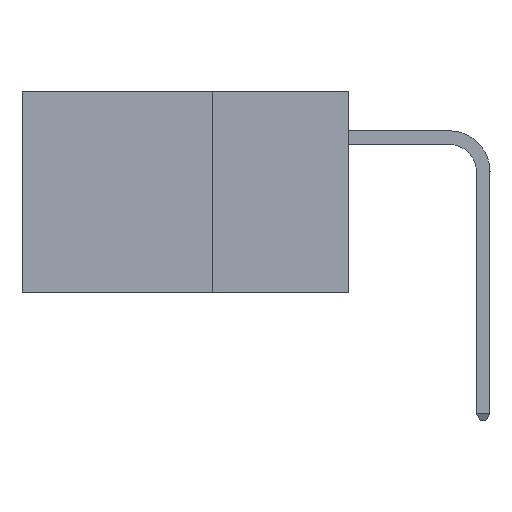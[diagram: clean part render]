
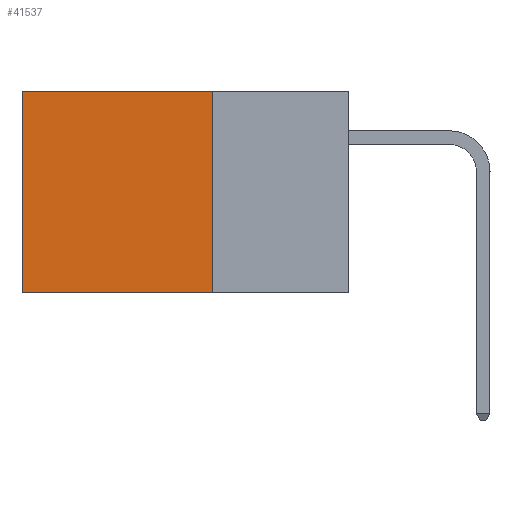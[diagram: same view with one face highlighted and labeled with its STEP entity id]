
A CAD part, left-side view. The second image highlights one B-rep face of the part: STEP entity #41537.
In plain terms, the highlighted planar face has unit normal (-1, 0, 0).
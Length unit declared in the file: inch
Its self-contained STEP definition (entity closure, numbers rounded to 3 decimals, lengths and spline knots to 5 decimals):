
#306 = ORIENTED_EDGE ( 'NONE', *, *, #25987, .F. ) ;
#321 = EDGE_CURVE ( 'NONE', #9929, #9612, #21247, .T. ) ;
#1148 = CARTESIAN_POINT ( 'NONE',  ( 0.2875, 0.25, 0. ) ) ;
#2748 = CARTESIAN_POINT ( 'NONE',  ( 0.2875, 0.6, 0. ) ) ;
#3598 = FACE_OUTER_BOUND ( 'NONE', #4497, .T. ) ;
#4399 = LINE ( 'NONE', #32380, #9884 ) ;
#4497 = EDGE_LOOP ( 'NONE', ( #27915, #306, #9105, #9770 ) ) ;
#5190 = CARTESIAN_POINT ( 'NONE',  ( 0.2875, 0.6, -0.37 ) ) ;
#6873 = VERTEX_POINT ( 'NONE', #39165 ) ;
#7708 = DIRECTION ( 'NONE',  ( 0., 0., -1. ) ) ;
#9105 = ORIENTED_EDGE ( 'NONE', *, *, #31277, .F. ) ;
#9612 = VERTEX_POINT ( 'NONE', #5190 ) ;
#9770 = ORIENTED_EDGE ( 'NONE', *, *, #43562, .T. ) ;
#9884 = VECTOR ( 'NONE', #39561, 39.37008 ) ;
#9929 = VERTEX_POINT ( 'NONE', #41348 ) ;
#13336 = VECTOR ( 'NONE', #37983, 39.37008 ) ;
#14070 = DIRECTION ( 'NONE',  ( 0., 0., -1. ) ) ;
#14296 = VECTOR ( 'NONE', #19797, 39.37008 ) ;
#14437 = PLANE ( 'NONE',  #30230 ) ;
#16466 = LINE ( 'NONE', #40562, #14296 ) ;
#18395 = DIRECTION ( 'NONE',  ( 1., 0., 0. ) ) ;
#19152 = VERTEX_POINT ( 'NONE', #22249 ) ;
#19797 = DIRECTION ( 'NONE',  ( 0., 1., 0. ) ) ;
#21247 = LINE ( 'NONE', #2748, #40940 ) ;
#22249 = CARTESIAN_POINT ( 'NONE',  ( 0.2875, 0.25, 0. ) ) ;
#25987 = EDGE_CURVE ( 'NONE', #6873, #9612, #4399, .T. ) ;
#27915 = ORIENTED_EDGE ( 'NONE', *, *, #321, .T. ) ;
#28627 = LINE ( 'NONE', #34462, #13336 ) ;
#30230 = AXIS2_PLACEMENT_3D ( 'NONE', #1148, #18395, #7708 ) ;
#31277 = EDGE_CURVE ( 'NONE', #19152, #6873, #28627, .T. ) ;
#32380 = CARTESIAN_POINT ( 'NONE',  ( 0.2875, 0.25, -0.37 ) ) ;
#34462 = CARTESIAN_POINT ( 'NONE',  ( 0.2875, 0.25, 0. ) ) ;
#37983 = DIRECTION ( 'NONE',  ( 0., 0., -1. ) ) ;
#39165 = CARTESIAN_POINT ( 'NONE',  ( 0.2875, 0.25, -0.37 ) ) ;
#39561 = DIRECTION ( 'NONE',  ( 0., 1., 0. ) ) ;
#40562 = CARTESIAN_POINT ( 'NONE',  ( 0.2875, 0.25, 0. ) ) ;
#40940 = VECTOR ( 'NONE', #14070, 39.37008 ) ;
#41348 = CARTESIAN_POINT ( 'NONE',  ( 0.2875, 0.6, 0. ) ) ;
#41537 = ADVANCED_FACE ( 'NONE', ( #3598 ), #14437, .F. ) ;
#43562 = EDGE_CURVE ( 'NONE', #19152, #9929, #16466, .T. ) ;
